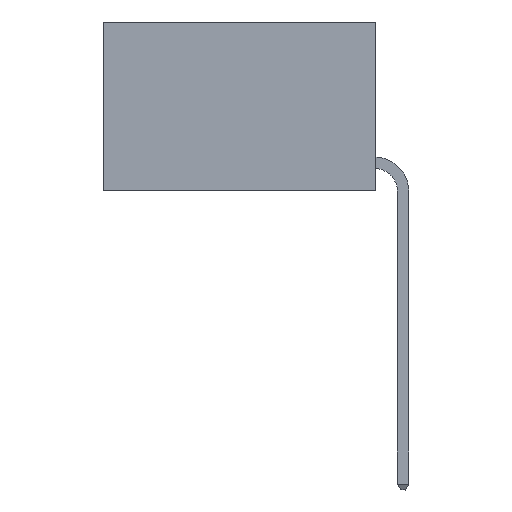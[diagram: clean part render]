
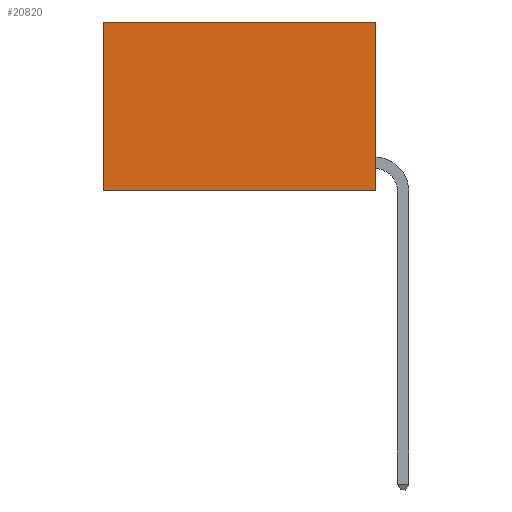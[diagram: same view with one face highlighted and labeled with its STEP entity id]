
A CAD part, left-side view. The second image highlights one B-rep face of the part: STEP entity #20820.
In plain terms, the highlighted planar face has unit normal (-1, 0, 0).
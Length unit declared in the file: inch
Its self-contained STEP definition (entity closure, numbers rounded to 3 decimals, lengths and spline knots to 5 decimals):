
#2044 = CARTESIAN_POINT ( 'NONE',  ( 0.2625, 0., 0. ) ) ;
#4466 = CARTESIAN_POINT ( 'NONE',  ( 0.2625, 0., -0.37 ) ) ;
#5705 = CARTESIAN_POINT ( 'NONE',  ( 0.2625, 0., 0. ) ) ;
#5765 = LINE ( 'NONE', #4466, #17254 ) ;
#5804 = CARTESIAN_POINT ( 'NONE',  ( 0.2625, 0.6, 0. ) ) ;
#6402 = ORIENTED_EDGE ( 'NONE', *, *, #24197, .F. ) ;
#6677 = DIRECTION ( 'NONE',  ( 1., 0., 0. ) ) ;
#8324 = EDGE_CURVE ( 'NONE', #23900, #9318, #5765, .T. ) ;
#8531 = CARTESIAN_POINT ( 'NONE',  ( 0.2625, 0., 0. ) ) ;
#9278 = CARTESIAN_POINT ( 'NONE',  ( 0.2625, 0., 0. ) ) ;
#9318 = VERTEX_POINT ( 'NONE', #21205 ) ;
#10390 = EDGE_LOOP ( 'NONE', ( #11454, #26613, #6402, #16802 ) ) ;
#10407 = VECTOR ( 'NONE', #15478, 39.37008 ) ;
#11198 = PLANE ( 'NONE',  #21315 ) ;
#11454 = ORIENTED_EDGE ( 'NONE', *, *, #25990, .T. ) ;
#11671 = CARTESIAN_POINT ( 'NONE',  ( 0.2625, 0., -0.37 ) ) ;
#12503 = DIRECTION ( 'NONE',  ( 0., 0., -1. ) ) ;
#12945 = LINE ( 'NONE', #5705, #29245 ) ;
#13326 = EDGE_CURVE ( 'NONE', #19900, #27834, #23103, .T. ) ;
#15478 = DIRECTION ( 'NONE',  ( 0., 1., 0. ) ) ;
#16802 = ORIENTED_EDGE ( 'NONE', *, *, #13326, .T. ) ;
#17130 = VECTOR ( 'NONE', #12503, 39.37008 ) ;
#17254 = VECTOR ( 'NONE', #29154, 39.37008 ) ;
#19900 = VERTEX_POINT ( 'NONE', #9278 ) ;
#20075 = FACE_OUTER_BOUND ( 'NONE', #10390, .T. ) ;
#20820 = ADVANCED_FACE ( 'NONE', ( #20075 ), #11198, .F. ) ;
#21205 = CARTESIAN_POINT ( 'NONE',  ( 0.2625, 0.6, -0.37 ) ) ;
#21315 = AXIS2_PLACEMENT_3D ( 'NONE', #2044, #6677, #22512 ) ;
#22512 = DIRECTION ( 'NONE',  ( 0., 0., -1. ) ) ;
#23103 = LINE ( 'NONE', #8531, #10407 ) ;
#23606 = CARTESIAN_POINT ( 'NONE',  ( 0.2625, 0.6, 0. ) ) ;
#23669 = LINE ( 'NONE', #23606, #17130 ) ;
#23900 = VERTEX_POINT ( 'NONE', #11671 ) ;
#24197 = EDGE_CURVE ( 'NONE', #19900, #23900, #12945, .T. ) ;
#25990 = EDGE_CURVE ( 'NONE', #27834, #9318, #23669, .T. ) ;
#26613 = ORIENTED_EDGE ( 'NONE', *, *, #8324, .F. ) ;
#27834 = VERTEX_POINT ( 'NONE', #5804 ) ;
#28227 = DIRECTION ( 'NONE',  ( 0., 0., -1. ) ) ;
#29154 = DIRECTION ( 'NONE',  ( 0., 1., 0. ) ) ;
#29245 = VECTOR ( 'NONE', #28227, 39.37008 ) ;
